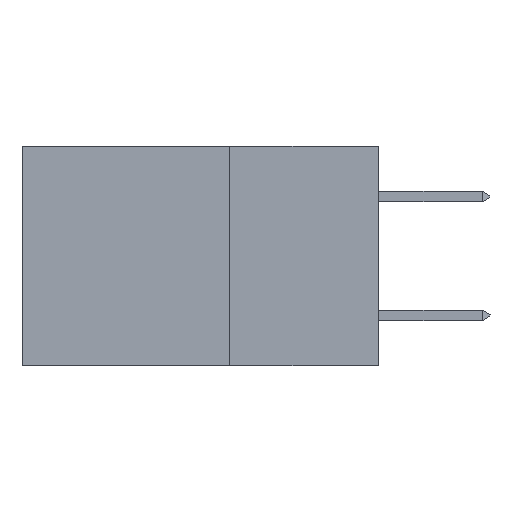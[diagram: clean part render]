
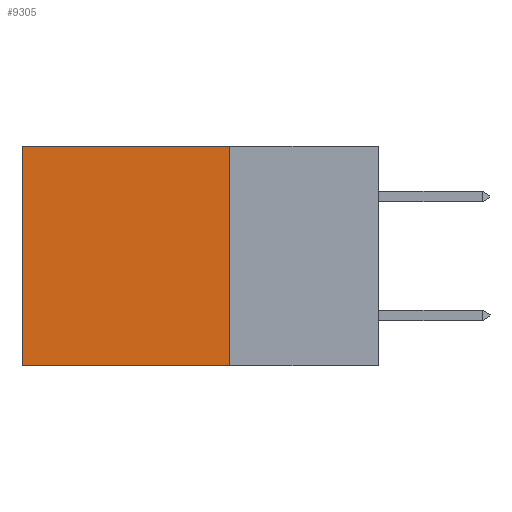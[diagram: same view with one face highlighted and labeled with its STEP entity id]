
A CAD part, left-side view. The second image highlights one B-rep face of the part: STEP entity #9305.
In plain terms, the highlighted planar face has unit normal (-1, 0, 0).
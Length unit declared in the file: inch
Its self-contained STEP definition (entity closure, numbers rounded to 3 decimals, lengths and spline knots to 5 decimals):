
#1133 = EDGE_CURVE ( 'NONE', #28059, #10468, #24708, .T. ) ;
#2461 = EDGE_CURVE ( 'NONE', #10468, #21051, #2628, .T. ) ;
#2628 = LINE ( 'NONE', #3743, #18437 ) ;
#3743 = CARTESIAN_POINT ( 'NONE',  ( 0.298, 0.6, 0. ) ) ;
#4092 = CARTESIAN_POINT ( 'NONE',  ( 0.298, 0.25, 0. ) ) ;
#4295 = DIRECTION ( 'NONE',  ( 0., 0., -1. ) ) ;
#6654 = CARTESIAN_POINT ( 'NONE',  ( 0.298, 0.25, 0. ) ) ;
#8011 = CARTESIAN_POINT ( 'NONE',  ( 0.298, 0.25, -0.37 ) ) ;
#8466 = CARTESIAN_POINT ( 'NONE',  ( 0.298, 0.6, 0. ) ) ;
#8922 = EDGE_LOOP ( 'NONE', ( #20977, #22818, #25182, #12545 ) ) ;
#9275 = VERTEX_POINT ( 'NONE', #25241 ) ;
#9305 = ADVANCED_FACE ( 'NONE', ( #10313 ), #30384, .F. ) ;
#10313 = FACE_OUTER_BOUND ( 'NONE', #8922, .T. ) ;
#10468 = VERTEX_POINT ( 'NONE', #8466 ) ;
#10842 = DIRECTION ( 'NONE',  ( 0., 0., -1. ) ) ;
#11695 = LINE ( 'NONE', #8011, #31325 ) ;
#12150 = EDGE_CURVE ( 'NONE', #9275, #21051, #11695, .T. ) ;
#12394 = VECTOR ( 'NONE', #24209, 39.37008 ) ;
#12545 = ORIENTED_EDGE ( 'NONE', *, *, #1133, .T. ) ;
#12890 = AXIS2_PLACEMENT_3D ( 'NONE', #18147, #25568, #10842 ) ;
#15069 = DIRECTION ( 'NONE',  ( 0., 1., 0. ) ) ;
#18147 = CARTESIAN_POINT ( 'NONE',  ( 0.298, 0.25, 0. ) ) ;
#18437 = VECTOR ( 'NONE', #4295, 39.37008 ) ;
#18987 = EDGE_CURVE ( 'NONE', #28059, #9275, #25399, .T. ) ;
#19612 = DIRECTION ( 'NONE',  ( 0., 0., -1. ) ) ;
#20977 = ORIENTED_EDGE ( 'NONE', *, *, #2461, .T. ) ;
#21051 = VERTEX_POINT ( 'NONE', #30285 ) ;
#22818 = ORIENTED_EDGE ( 'NONE', *, *, #12150, .F. ) ;
#24209 = DIRECTION ( 'NONE',  ( 0., 1., 0. ) ) ;
#24257 = VECTOR ( 'NONE', #19612, 39.37008 ) ;
#24382 = CARTESIAN_POINT ( 'NONE',  ( 0.298, 0.25, 0. ) ) ;
#24708 = LINE ( 'NONE', #6654, #12394 ) ;
#25182 = ORIENTED_EDGE ( 'NONE', *, *, #18987, .F. ) ;
#25241 = CARTESIAN_POINT ( 'NONE',  ( 0.298, 0.25, -0.37 ) ) ;
#25399 = LINE ( 'NONE', #4092, #24257 ) ;
#25568 = DIRECTION ( 'NONE',  ( 1., 0., 0. ) ) ;
#28059 = VERTEX_POINT ( 'NONE', #24382 ) ;
#30285 = CARTESIAN_POINT ( 'NONE',  ( 0.298, 0.6, -0.37 ) ) ;
#30384 = PLANE ( 'NONE',  #12890 ) ;
#31325 = VECTOR ( 'NONE', #15069, 39.37008 ) ;
